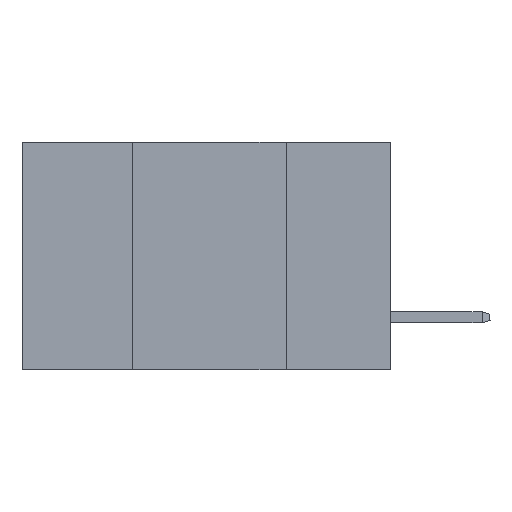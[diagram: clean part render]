
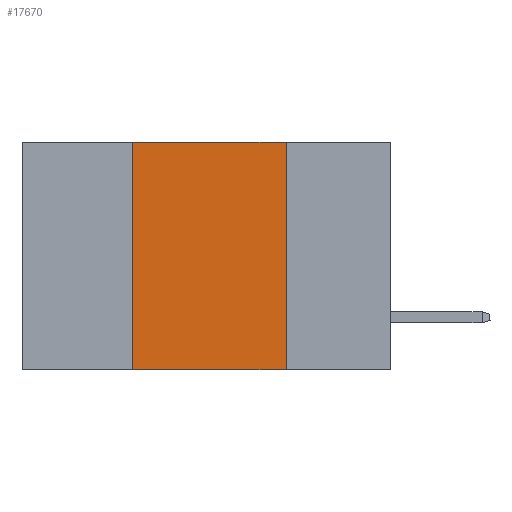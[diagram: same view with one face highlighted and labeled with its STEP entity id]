
A CAD part, left-side view. The second image highlights one B-rep face of the part: STEP entity #17670.
In plain terms, the highlighted planar face has unit normal (-1, 0, 0).
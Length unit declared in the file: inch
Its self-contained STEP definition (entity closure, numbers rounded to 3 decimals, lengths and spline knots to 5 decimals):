
#253 = LINE ( 'NONE', #4756, #14158 ) ;
#478 = DIRECTION ( 'NONE',  ( 0., 0., 1. ) ) ;
#2070 = DIRECTION ( 'NONE',  ( 0., -1., 0. ) ) ;
#2325 = CARTESIAN_POINT ( 'NONE',  ( 0., 0.17, 0. ) ) ;
#2362 = ORIENTED_EDGE ( 'NONE', *, *, #10860, .T. ) ;
#2425 = LINE ( 'NONE', #7864, #3033 ) ;
#3033 = VECTOR ( 'NONE', #15051, 39.37008 ) ;
#3373 = PLANE ( 'NONE',  #5613 ) ;
#3617 = CARTESIAN_POINT ( 'NONE',  ( 0., 0.42, -0.37 ) ) ;
#3691 = FACE_OUTER_BOUND ( 'NONE', #9220, .T. ) ;
#4241 = ORIENTED_EDGE ( 'NONE', *, *, #13437, .F. ) ;
#4756 = CARTESIAN_POINT ( 'NONE',  ( 0., 0.42, 0. ) ) ;
#5025 = VERTEX_POINT ( 'NONE', #3617 ) ;
#5613 = AXIS2_PLACEMENT_3D ( 'NONE', #15021, #15404, #14064 ) ;
#5721 = EDGE_CURVE ( 'NONE', #5025, #17108, #253, .T. ) ;
#6053 = CARTESIAN_POINT ( 'NONE',  ( 0., 0.42, 0. ) ) ;
#7187 = VECTOR ( 'NONE', #2070, 39.37008 ) ;
#7516 = VECTOR ( 'NONE', #16968, 39.37008 ) ;
#7845 = CARTESIAN_POINT ( 'NONE',  ( 0., 0.6, -0.37 ) ) ;
#7864 = CARTESIAN_POINT ( 'NONE',  ( 0., 0.6, 0. ) ) ;
#8325 = EDGE_CURVE ( 'NONE', #12915, #13754, #14567, .T. ) ;
#9220 = EDGE_LOOP ( 'NONE', ( #11986, #4241, #17672, #2362 ) ) ;
#10860 = EDGE_CURVE ( 'NONE', #5025, #13754, #17438, .T. ) ;
#11047 = CARTESIAN_POINT ( 'NONE',  ( 0., 0.17, 0. ) ) ;
#11986 = ORIENTED_EDGE ( 'NONE', *, *, #8325, .F. ) ;
#12915 = VERTEX_POINT ( 'NONE', #11047 ) ;
#13263 = CARTESIAN_POINT ( 'NONE',  ( 0., 0.17, -0.37 ) ) ;
#13437 = EDGE_CURVE ( 'NONE', #17108, #12915, #2425, .T. ) ;
#13754 = VERTEX_POINT ( 'NONE', #13263 ) ;
#14064 = DIRECTION ( 'NONE',  ( 0., 0., -1. ) ) ;
#14158 = VECTOR ( 'NONE', #478, 39.37008 ) ;
#14567 = LINE ( 'NONE', #2325, #7516 ) ;
#15021 = CARTESIAN_POINT ( 'NONE',  ( 0., 0.6, 0. ) ) ;
#15051 = DIRECTION ( 'NONE',  ( 0., -1., 0. ) ) ;
#15404 = DIRECTION ( 'NONE',  ( 1., 0., 0. ) ) ;
#16968 = DIRECTION ( 'NONE',  ( 0., 0., -1. ) ) ;
#17108 = VERTEX_POINT ( 'NONE', #6053 ) ;
#17438 = LINE ( 'NONE', #7845, #7187 ) ;
#17670 = ADVANCED_FACE ( 'NONE', ( #3691 ), #3373, .F. ) ;
#17672 = ORIENTED_EDGE ( 'NONE', *, *, #5721, .F. ) ;
